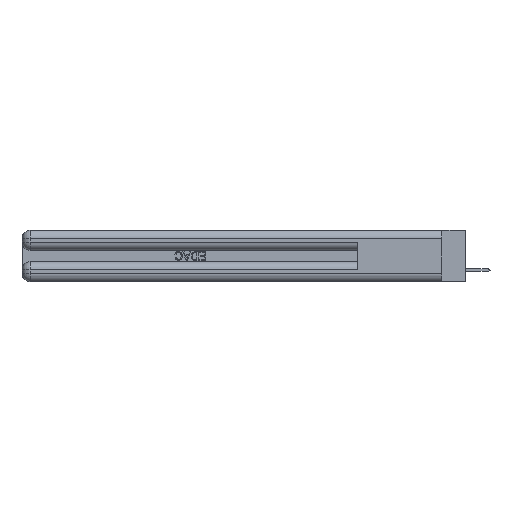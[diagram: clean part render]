
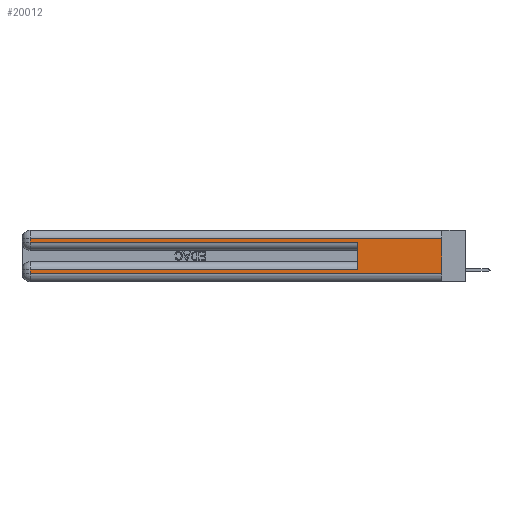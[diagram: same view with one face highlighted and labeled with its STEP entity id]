
A CAD part, left-side view. The second image highlights one B-rep face of the part: STEP entity #20012.
In plain terms, the highlighted planar face has unit normal (-1, 0, 0).
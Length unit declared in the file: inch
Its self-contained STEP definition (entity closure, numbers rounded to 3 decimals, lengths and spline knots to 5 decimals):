
#914 = VERTEX_POINT ( 'NONE', #48339 ) ;
#1018 = CARTESIAN_POINT ( 'NONE',  ( 0., 2.94, 0.37 ) ) ;
#1531 = CARTESIAN_POINT ( 'NONE',  ( 0., 2.94, 0.285 ) ) ;
#1604 = EDGE_CURVE ( 'NONE', #39233, #12091, #13870, .T. ) ;
#2243 = DIRECTION ( 'NONE',  ( 0., 0., -1. ) ) ;
#3403 = VECTOR ( 'NONE', #36149, 39.37008 ) ;
#3685 = DIRECTION ( 'NONE',  ( 0., 1., 0. ) ) ;
#7269 = ORIENTED_EDGE ( 'NONE', *, *, #46404, .T. ) ;
#7364 = CARTESIAN_POINT ( 'NONE',  ( 0., 2.94, 0.37 ) ) ;
#8459 = CARTESIAN_POINT ( 'NONE',  ( 0., 2.94, 0.085 ) ) ;
#9927 = VECTOR ( 'NONE', #3685, 39.37008 ) ;
#11089 = CARTESIAN_POINT ( 'NONE',  ( 0., 0.6, 0.085 ) ) ;
#11107 = CARTESIAN_POINT ( 'NONE',  ( 0., 0., 0.31 ) ) ;
#12032 = DIRECTION ( 'NONE',  ( 0., 0., -1. ) ) ;
#12091 = VERTEX_POINT ( 'NONE', #8459 ) ;
#12479 = EDGE_LOOP ( 'NONE', ( #26344, #14444, #7269, #30902, #14273, #39876, #23671, #30359 ) ) ;
#13153 = EDGE_CURVE ( 'NONE', #36050, #914, #29595, .T. ) ;
#13870 = LINE ( 'NONE', #37233, #18582 ) ;
#14273 = ORIENTED_EDGE ( 'NONE', *, *, #22902, .F. ) ;
#14444 = ORIENTED_EDGE ( 'NONE', *, *, #36022, .T. ) ;
#14721 = LINE ( 'NONE', #39342, #31188 ) ;
#18236 = CARTESIAN_POINT ( 'NONE',  ( 0., 2.94, 0.06 ) ) ;
#18406 = DIRECTION ( 'NONE',  ( 0., 1., 0. ) ) ;
#18582 = VECTOR ( 'NONE', #18406, 39.37008 ) ;
#18818 = CARTESIAN_POINT ( 'NONE',  ( 0., 2.94, 0.31 ) ) ;
#20012 = ADVANCED_FACE ( 'NONE', ( #47324 ), #23469, .F. ) ;
#20613 = LINE ( 'NONE', #27117, #40116 ) ;
#22247 = LINE ( 'NONE', #7364, #22863 ) ;
#22863 = VECTOR ( 'NONE', #26449, 39.37008 ) ;
#22902 = EDGE_CURVE ( 'NONE', #39233, #24517, #20613, .T. ) ;
#23469 = PLANE ( 'NONE',  #37334 ) ;
#23633 = EDGE_CURVE ( 'NONE', #32984, #24517, #25852, .T. ) ;
#23671 = ORIENTED_EDGE ( 'NONE', *, *, #44173, .T. ) ;
#24517 = VERTEX_POINT ( 'NONE', #32403 ) ;
#25852 = LINE ( 'NONE', #28037, #3403 ) ;
#26344 = ORIENTED_EDGE ( 'NONE', *, *, #43750, .F. ) ;
#26449 = DIRECTION ( 'NONE',  ( 0., 0., -1. ) ) ;
#27117 = CARTESIAN_POINT ( 'NONE',  ( 0., 0.6, 0.145 ) ) ;
#28037 = CARTESIAN_POINT ( 'NONE',  ( 0., 0., 0.285 ) ) ;
#29551 = CARTESIAN_POINT ( 'NONE',  ( 0., 0., 0.31 ) ) ;
#29595 = LINE ( 'NONE', #32989, #41336 ) ;
#30359 = ORIENTED_EDGE ( 'NONE', *, *, #13153, .T. ) ;
#30902 = ORIENTED_EDGE ( 'NONE', *, *, #23633, .T. ) ;
#31188 = VECTOR ( 'NONE', #2243, 39.37008 ) ;
#31214 = VECTOR ( 'NONE', #12032, 39.37008 ) ;
#31361 = DIRECTION ( 'NONE',  ( 1., 0., 0. ) ) ;
#32403 = CARTESIAN_POINT ( 'NONE',  ( 0., 0.6, 0.285 ) ) ;
#32984 = VERTEX_POINT ( 'NONE', #1531 ) ;
#32989 = CARTESIAN_POINT ( 'NONE',  ( 0., 0., 0.06 ) ) ;
#33313 = VERTEX_POINT ( 'NONE', #18818 ) ;
#36022 = EDGE_CURVE ( 'NONE', #47003, #33313, #40001, .T. ) ;
#36050 = VERTEX_POINT ( 'NONE', #18236 ) ;
#36149 = DIRECTION ( 'NONE',  ( 0., -1., 0. ) ) ;
#37233 = CARTESIAN_POINT ( 'NONE',  ( 0., 0., 0.085 ) ) ;
#37334 = AXIS2_PLACEMENT_3D ( 'NONE', #38453, #31361, #38781 ) ;
#38453 = CARTESIAN_POINT ( 'NONE',  ( 0., 0., 0.37 ) ) ;
#38500 = DIRECTION ( 'NONE',  ( 0., 0., 1. ) ) ;
#38781 = DIRECTION ( 'NONE',  ( 0., 0., -1. ) ) ;
#39233 = VERTEX_POINT ( 'NONE', #11089 ) ;
#39342 = CARTESIAN_POINT ( 'NONE',  ( 0., 0., 0.37 ) ) ;
#39876 = ORIENTED_EDGE ( 'NONE', *, *, #1604, .T. ) ;
#40001 = LINE ( 'NONE', #11107, #9927 ) ;
#40116 = VECTOR ( 'NONE', #38500, 39.37008 ) ;
#41336 = VECTOR ( 'NONE', #48239, 39.37008 ) ;
#41562 = LINE ( 'NONE', #1018, #31214 ) ;
#43750 = EDGE_CURVE ( 'NONE', #47003, #914, #14721, .T. ) ;
#44173 = EDGE_CURVE ( 'NONE', #12091, #36050, #41562, .T. ) ;
#46404 = EDGE_CURVE ( 'NONE', #33313, #32984, #22247, .T. ) ;
#47003 = VERTEX_POINT ( 'NONE', #29551 ) ;
#47324 = FACE_OUTER_BOUND ( 'NONE', #12479, .T. ) ;
#48239 = DIRECTION ( 'NONE',  ( 0., -1., 0. ) ) ;
#48339 = CARTESIAN_POINT ( 'NONE',  ( 0., 0., 0.06 ) ) ;
